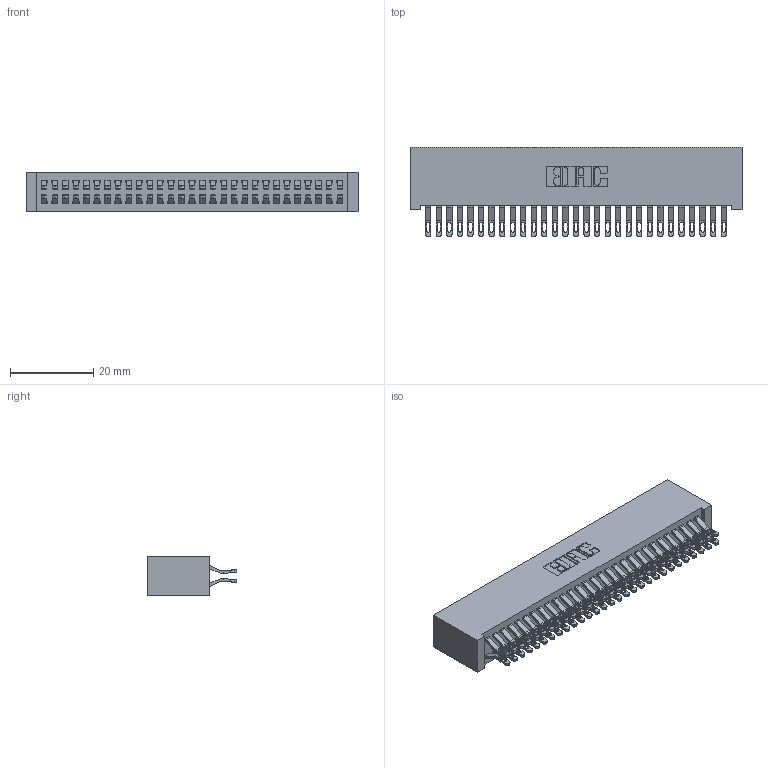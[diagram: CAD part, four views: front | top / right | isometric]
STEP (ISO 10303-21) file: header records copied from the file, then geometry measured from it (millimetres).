
FILE_DESCRIPTION (( 'STEP AP203' ), '1' );
FILE_NAME ('392-058-555-201.STEP', '2019-10-08T16:51:07', ( '' ), ( '' ), 'SwSTEP 2.0', 'SolidWorks 2016', '' );
FILE_SCHEMA (( 'CONFIG_CONTROL_DESIGN' ));
Length unit declared in the file: inch
Products named in the file (3): 345-292-001_555 Tail; 392-058-555-201; 342 Part_Lugless
Assembly tree (59 placements, depth 2):
  392-058-555-201
    342 Part_Lugless
    345-292-001_555 Tail  x58
Bounding box: 79.91 x 21.47 x 9.4 mm (x, y, z)
Volume: 7718.9 mm3; surface area: 13251.6 mm2
Topology: 59 solids, 59 shells, 3466 faces, 10889 edges, 7258 vertices
Faces by surface type: plane 2034, cylinder 1432
Entity records: 20255 total; most frequent: CARTESIAN_POINT 3404, ORIENTED_EDGE 3310, DIRECTION 2895, EDGE_CURVE 1655, LINE 1515, VECTOR 1515, VERTEX_POINT 1102, AXIS2_PLACEMENT_3D 690
